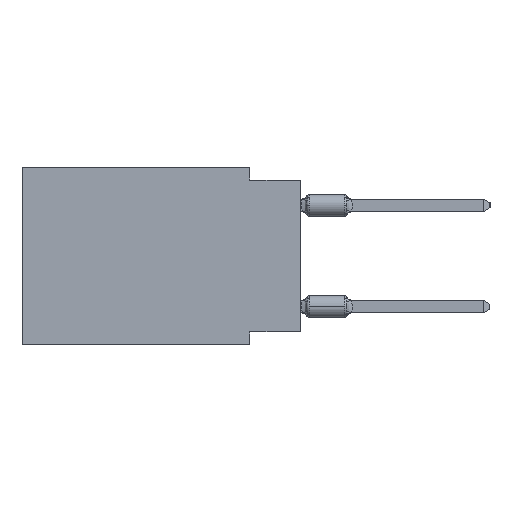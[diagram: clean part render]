
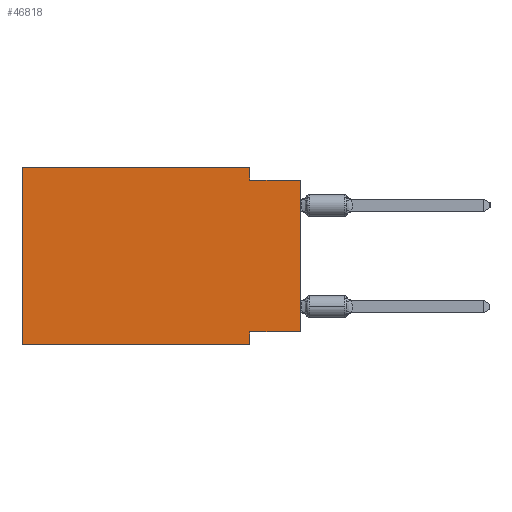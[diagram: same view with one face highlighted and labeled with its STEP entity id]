
A CAD part, left-side view. The second image highlights one B-rep face of the part: STEP entity #46818.
In plain terms, the highlighted planar face has unit normal (-1, 0, 0).
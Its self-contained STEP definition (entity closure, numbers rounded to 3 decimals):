
#561 = DIRECTION ( 'NONE',  ( 0., -1., 0. ) ) ;
#834 = DIRECTION ( 'NONE',  ( 0., 0., -1. ) ) ;
#946 = VECTOR ( 'NONE', #3471, 1000. ) ;
#1887 = DIRECTION ( 'NONE',  ( 0., 1., 0. ) ) ;
#2137 = CARTESIAN_POINT ( 'NONE',  ( 0., 0., -8.255 ) ) ;
#2956 = CARTESIAN_POINT ( 'NONE',  ( 0., 13.97, 0. ) ) ;
#3169 = CARTESIAN_POINT ( 'NONE',  ( 0., 0., -0.635 ) ) ;
#3356 = DIRECTION ( 'NONE',  ( 0., -1., 0. ) ) ;
#3471 = DIRECTION ( 'NONE',  ( 0., 0., 1. ) ) ;
#4332 = ORIENTED_EDGE ( 'NONE', *, *, #45597, .F. ) ;
#4373 = CARTESIAN_POINT ( 'NONE',  ( 0., 13.97, 0. ) ) ;
#4715 = EDGE_CURVE ( 'NONE', #10077, #18383, #31470, .T. ) ;
#4739 = CARTESIAN_POINT ( 'NONE',  ( 0., 2.54, -8.255 ) ) ;
#4923 = CARTESIAN_POINT ( 'NONE',  ( 0., 0., -0.635 ) ) ;
#5540 = CARTESIAN_POINT ( 'NONE',  ( 0., 2.54, -0.635 ) ) ;
#5582 = VERTEX_POINT ( 'NONE', #23726 ) ;
#5826 = CARTESIAN_POINT ( 'NONE',  ( 0., 2.54, -8.89 ) ) ;
#6159 = DIRECTION ( 'NONE',  ( 0., 0., -1. ) ) ;
#6463 = AXIS2_PLACEMENT_3D ( 'NONE', #4373, #32234, #48117 ) ;
#8466 = EDGE_CURVE ( 'NONE', #10077, #26660, #31849, .T. ) ;
#8729 = VERTEX_POINT ( 'NONE', #5540 ) ;
#10077 = VERTEX_POINT ( 'NONE', #42387 ) ;
#10445 = VECTOR ( 'NONE', #46157, 1000. ) ;
#11029 = LINE ( 'NONE', #3169, #10445 ) ;
#11630 = CARTESIAN_POINT ( 'NONE',  ( 0., 13.97, 0. ) ) ;
#16752 = EDGE_CURVE ( 'NONE', #24137, #25537, #33670, .T. ) ;
#18082 = VECTOR ( 'NONE', #1887, 1000. ) ;
#18359 = ORIENTED_EDGE ( 'NONE', *, *, #4715, .T. ) ;
#18383 = VERTEX_POINT ( 'NONE', #5826 ) ;
#18828 = ORIENTED_EDGE ( 'NONE', *, *, #16752, .F. ) ;
#20590 = ORIENTED_EDGE ( 'NONE', *, *, #21767, .F. ) ;
#21767 = EDGE_CURVE ( 'NONE', #8729, #22470, #11029, .T. ) ;
#22470 = VERTEX_POINT ( 'NONE', #4923 ) ;
#23726 = CARTESIAN_POINT ( 'NONE',  ( 0., 2.54, 0. ) ) ;
#24137 = VERTEX_POINT ( 'NONE', #42249 ) ;
#24156 = PLANE ( 'NONE',  #6463 ) ;
#24951 = EDGE_LOOP ( 'NONE', ( #43842, #20590, #4332, #35831, #30035, #18359, #33482, #18828 ) ) ;
#25315 = CARTESIAN_POINT ( 'NONE',  ( 0., 2.54, -8.89 ) ) ;
#25494 = EDGE_CURVE ( 'NONE', #26660, #5582, #39193, .T. ) ;
#25537 = VERTEX_POINT ( 'NONE', #4739 ) ;
#26660 = VERTEX_POINT ( 'NONE', #11630 ) ;
#27528 = VECTOR ( 'NONE', #31644, 1000. ) ;
#28001 = VECTOR ( 'NONE', #561, 1000. ) ;
#28059 = FACE_OUTER_BOUND ( 'NONE', #24951, .T. ) ;
#29954 = VECTOR ( 'NONE', #3356, 1000. ) ;
#30035 = ORIENTED_EDGE ( 'NONE', *, *, #8466, .F. ) ;
#31470 = LINE ( 'NONE', #35367, #29954 ) ;
#31644 = DIRECTION ( 'NONE',  ( 0., 0., 1. ) ) ;
#31849 = LINE ( 'NONE', #2956, #946 ) ;
#32234 = DIRECTION ( 'NONE',  ( 1., 0., 0. ) ) ;
#32514 = VECTOR ( 'NONE', #6159, 1000. ) ;
#33482 = ORIENTED_EDGE ( 'NONE', *, *, #38616, .F. ) ;
#33670 = LINE ( 'NONE', #2137, #18082 ) ;
#35279 = LINE ( 'NONE', #51173, #27528 ) ;
#35367 = CARTESIAN_POINT ( 'NONE',  ( 0., 13.97, -8.89 ) ) ;
#35831 = ORIENTED_EDGE ( 'NONE', *, *, #25494, .F. ) ;
#36773 = LINE ( 'NONE', #25315, #48566 ) ;
#38616 = EDGE_CURVE ( 'NONE', #25537, #18383, #36773, .T. ) ;
#38936 = CARTESIAN_POINT ( 'NONE',  ( 0., 13.97, 0. ) ) ;
#39193 = LINE ( 'NONE', #38936, #28001 ) ;
#42249 = CARTESIAN_POINT ( 'NONE',  ( 0., 0., -8.255 ) ) ;
#42387 = CARTESIAN_POINT ( 'NONE',  ( 0., 13.97, -8.89 ) ) ;
#43842 = ORIENTED_EDGE ( 'NONE', *, *, #45884, .T. ) ;
#44984 = LINE ( 'NONE', #48887, #32514 ) ;
#45597 = EDGE_CURVE ( 'NONE', #5582, #8729, #44984, .T. ) ;
#45884 = EDGE_CURVE ( 'NONE', #24137, #22470, #35279, .T. ) ;
#46157 = DIRECTION ( 'NONE',  ( 0., -1., 0. ) ) ;
#46818 = ADVANCED_FACE ( 'NONE', ( #28059 ), #24156, .F. ) ;
#48117 = DIRECTION ( 'NONE',  ( 0., 0., -1. ) ) ;
#48566 = VECTOR ( 'NONE', #834, 1000. ) ;
#48887 = CARTESIAN_POINT ( 'NONE',  ( 0., 2.54, 0. ) ) ;
#51173 = CARTESIAN_POINT ( 'NONE',  ( 0., 0., 0. ) ) ;
